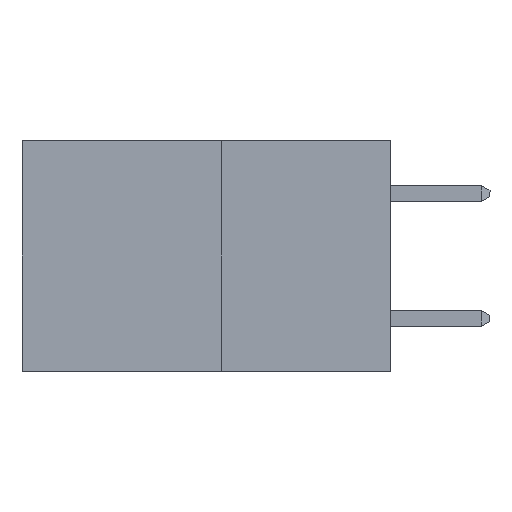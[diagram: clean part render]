
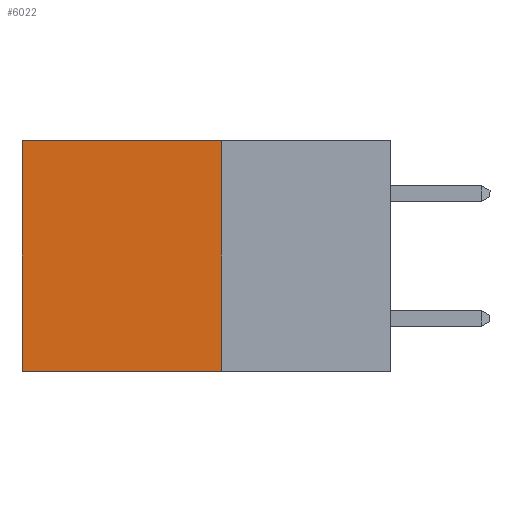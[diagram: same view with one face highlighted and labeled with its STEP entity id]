
A CAD part, left-side view. The second image highlights one B-rep face of the part: STEP entity #6022.
In plain terms, the highlighted planar face has unit normal (-1, 0, 0).
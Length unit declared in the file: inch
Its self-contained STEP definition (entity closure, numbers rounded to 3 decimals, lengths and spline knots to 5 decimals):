
#224 = ORIENTED_EDGE ( 'NONE', *, *, #509, .F. ) ;
#483 = ORIENTED_EDGE ( 'NONE', *, *, #7062, .T. ) ;
#509 = EDGE_CURVE ( 'NONE', #5719, #2560, #3228, .T. ) ;
#746 = ORIENTED_EDGE ( 'NONE', *, *, #7774, .T. ) ;
#1156 = FACE_OUTER_BOUND ( 'NONE', #2974, .T. ) ;
#1349 = VECTOR ( 'NONE', #6037, 39.37008 ) ;
#1692 = VECTOR ( 'NONE', #3873, 39.37008 ) ;
#2420 = DIRECTION ( 'NONE',  ( 0., 0., -1. ) ) ;
#2435 = DIRECTION ( 'NONE',  ( 1., 0., 0. ) ) ;
#2560 = VERTEX_POINT ( 'NONE', #7682 ) ;
#2625 = CARTESIAN_POINT ( 'NONE',  ( 0.277, 0.27, -0.37 ) ) ;
#2672 = PLANE ( 'NONE',  #8106 ) ;
#2974 = EDGE_LOOP ( 'NONE', ( #483, #6531, #224, #746 ) ) ;
#3228 = LINE ( 'NONE', #6971, #4687 ) ;
#3278 = LINE ( 'NONE', #3887, #1692 ) ;
#3873 = DIRECTION ( 'NONE',  ( 0., 1., 0. ) ) ;
#3887 = CARTESIAN_POINT ( 'NONE',  ( 0.277, 0.27, 0. ) ) ;
#4294 = EDGE_CURVE ( 'NONE', #2560, #4585, #4873, .T. ) ;
#4585 = VERTEX_POINT ( 'NONE', #8205 ) ;
#4653 = LINE ( 'NONE', #6065, #1349 ) ;
#4687 = VECTOR ( 'NONE', #5344, 39.37008 ) ;
#4873 = LINE ( 'NONE', #7497, #6411 ) ;
#5344 = DIRECTION ( 'NONE',  ( 0., 0., -1. ) ) ;
#5570 = VERTEX_POINT ( 'NONE', #7687 ) ;
#5608 = CARTESIAN_POINT ( 'NONE',  ( 0.277, 0.27, 0. ) ) ;
#5719 = VERTEX_POINT ( 'NONE', #5608 ) ;
#6022 = ADVANCED_FACE ( 'NONE', ( #1156 ), #2672, .F. ) ;
#6037 = DIRECTION ( 'NONE',  ( 0., 0., -1. ) ) ;
#6065 = CARTESIAN_POINT ( 'NONE',  ( 0.277, 0.59, -0.37 ) ) ;
#6411 = VECTOR ( 'NONE', #7327, 39.37008 ) ;
#6531 = ORIENTED_EDGE ( 'NONE', *, *, #4294, .F. ) ;
#6971 = CARTESIAN_POINT ( 'NONE',  ( 0.277, 0.27, -0.37 ) ) ;
#7062 = EDGE_CURVE ( 'NONE', #5570, #4585, #4653, .T. ) ;
#7327 = DIRECTION ( 'NONE',  ( 0., 1., 0. ) ) ;
#7497 = CARTESIAN_POINT ( 'NONE',  ( 0.277, 0.27, -0.37 ) ) ;
#7682 = CARTESIAN_POINT ( 'NONE',  ( 0.277, 0.27, -0.37 ) ) ;
#7687 = CARTESIAN_POINT ( 'NONE',  ( 0.277, 0.59, 0. ) ) ;
#7774 = EDGE_CURVE ( 'NONE', #5719, #5570, #3278, .T. ) ;
#8106 = AXIS2_PLACEMENT_3D ( 'NONE', #2625, #2435, #2420 ) ;
#8205 = CARTESIAN_POINT ( 'NONE',  ( 0.277, 0.59, -0.37 ) ) ;
